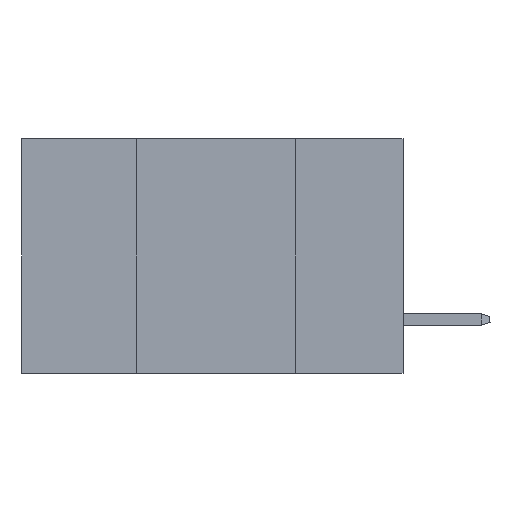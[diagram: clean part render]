
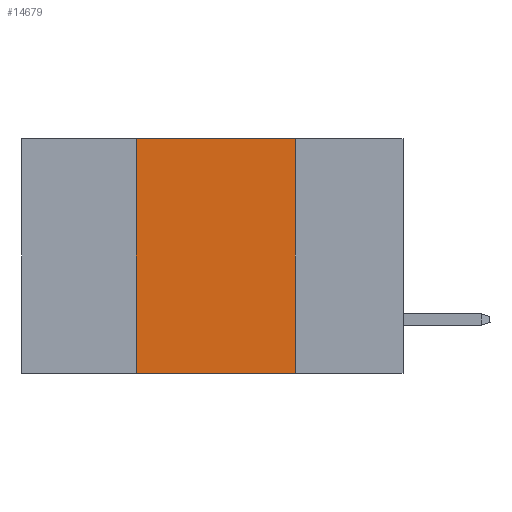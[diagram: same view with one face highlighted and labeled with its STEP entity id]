
A CAD part, left-side view. The second image highlights one B-rep face of the part: STEP entity #14679.
In plain terms, the highlighted planar face has unit normal (-1, 0, 0).
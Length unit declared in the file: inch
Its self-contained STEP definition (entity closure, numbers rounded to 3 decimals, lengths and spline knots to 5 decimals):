
#2082 = VERTEX_POINT ( 'NONE', #39365 ) ;
#3434 = LINE ( 'NONE', #37595, #30654 ) ;
#5988 = DIRECTION ( 'NONE',  ( 1., 0., 0. ) ) ;
#8945 = CARTESIAN_POINT ( 'NONE',  ( 0., 0.6, 0. ) ) ;
#9613 = FACE_OUTER_BOUND ( 'NONE', #25327, .T. ) ;
#10467 = EDGE_CURVE ( 'NONE', #22754, #24681, #3434, .T. ) ;
#11893 = ORIENTED_EDGE ( 'NONE', *, *, #12753, .T. ) ;
#12753 = EDGE_CURVE ( 'NONE', #22171, #24681, #44557, .T. ) ;
#13333 = CARTESIAN_POINT ( 'NONE',  ( 0., 0.6, -0.37 ) ) ;
#13557 = DIRECTION ( 'NONE',  ( 0., -1., 0. ) ) ;
#14679 = ADVANCED_FACE ( 'NONE', ( #9613 ), #36301, .F. ) ;
#16607 = CARTESIAN_POINT ( 'NONE',  ( 0., 0.42, 0. ) ) ;
#21212 = CARTESIAN_POINT ( 'NONE',  ( 0., 0.17, 0. ) ) ;
#22171 = VERTEX_POINT ( 'NONE', #26786 ) ;
#22175 = EDGE_CURVE ( 'NONE', #22171, #2082, #40586, .T. ) ;
#22475 = DIRECTION ( 'NONE',  ( 0., -1., 0. ) ) ;
#22754 = VERTEX_POINT ( 'NONE', #21212 ) ;
#24640 = ORIENTED_EDGE ( 'NONE', *, *, #22175, .F. ) ;
#24681 = VERTEX_POINT ( 'NONE', #38053 ) ;
#25327 = EDGE_LOOP ( 'NONE', ( #36514, #38402, #24640, #11893 ) ) ;
#26786 = CARTESIAN_POINT ( 'NONE',  ( 0., 0.42, -0.37 ) ) ;
#27213 = DIRECTION ( 'NONE',  ( 0., 0., -1. ) ) ;
#27728 = VECTOR ( 'NONE', #37179, 39.37008 ) ;
#30654 = VECTOR ( 'NONE', #27213, 39.37008 ) ;
#33367 = DIRECTION ( 'NONE',  ( 0., 0., -1. ) ) ;
#35580 = CARTESIAN_POINT ( 'NONE',  ( 0., 0.6, 0. ) ) ;
#36301 = PLANE ( 'NONE',  #41908 ) ;
#36514 = ORIENTED_EDGE ( 'NONE', *, *, #10467, .F. ) ;
#37179 = DIRECTION ( 'NONE',  ( 0., 0., 1. ) ) ;
#37595 = CARTESIAN_POINT ( 'NONE',  ( 0., 0.17, 0. ) ) ;
#38053 = CARTESIAN_POINT ( 'NONE',  ( 0., 0.17, -0.37 ) ) ;
#38402 = ORIENTED_EDGE ( 'NONE', *, *, #43473, .F. ) ;
#38978 = LINE ( 'NONE', #35580, #43626 ) ;
#39365 = CARTESIAN_POINT ( 'NONE',  ( 0., 0.42, 0. ) ) ;
#40586 = LINE ( 'NONE', #16607, #27728 ) ;
#41908 = AXIS2_PLACEMENT_3D ( 'NONE', #8945, #5988, #33367 ) ;
#43422 = VECTOR ( 'NONE', #13557, 39.37008 ) ;
#43473 = EDGE_CURVE ( 'NONE', #2082, #22754, #38978, .T. ) ;
#43626 = VECTOR ( 'NONE', #22475, 39.37008 ) ;
#44557 = LINE ( 'NONE', #13333, #43422 ) ;
